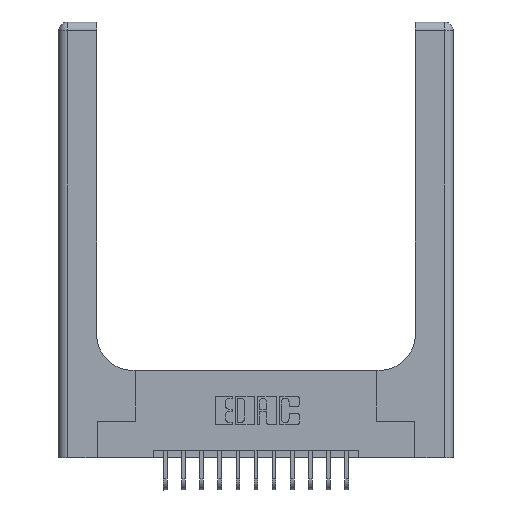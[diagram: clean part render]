
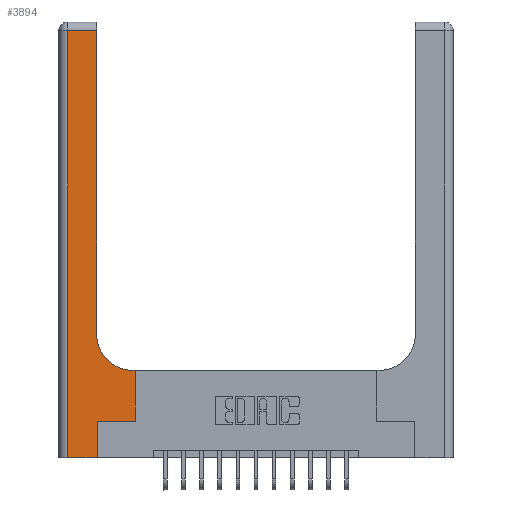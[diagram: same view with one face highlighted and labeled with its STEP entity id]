
A CAD part, top view. The second image highlights one B-rep face of the part: STEP entity #3894.
In plain terms, the highlighted planar face has unit normal (0, 0, 1).
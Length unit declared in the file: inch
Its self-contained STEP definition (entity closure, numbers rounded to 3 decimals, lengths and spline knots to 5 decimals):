
#65 = VECTOR ( 'NONE', #11523, 39.37008 ) ;
#504 = LINE ( 'NONE', #10790, #7117 ) ;
#634 = EDGE_LOOP ( 'NONE', ( #9870, #12955, #15927, #17325, #8818, #16133, #2347, #7431, #12916 ) ) ;
#816 = CARTESIAN_POINT ( 'NONE',  ( 0.06, 2.94, 0.37 ) ) ;
#871 = VECTOR ( 'NONE', #4851, 39.37008 ) ;
#942 = DIRECTION ( 'NONE',  ( 1., 0., 0. ) ) ;
#1199 = EDGE_CURVE ( 'NONE', #12617, #5967, #4763, .T. ) ;
#1299 = VECTOR ( 'NONE', #5661, 39.37008 ) ;
#1865 = DIRECTION ( 'NONE',  ( 0., 0., -1. ) ) ;
#1912 = VECTOR ( 'NONE', #942, 39.37008 ) ;
#2347 = ORIENTED_EDGE ( 'NONE', *, *, #17302, .T. ) ;
#2760 = CIRCLE ( 'NONE', #18224, 0.25 ) ;
#3000 = LINE ( 'NONE', #14559, #1299 ) ;
#3154 = CARTESIAN_POINT ( 'NONE',  ( 0.265, 0., 0.37 ) ) ;
#3252 = LINE ( 'NONE', #4483, #65 ) ;
#3894 = ADVANCED_FACE ( 'NONE', ( #18105 ), #4156, .F. ) ;
#4156 = PLANE ( 'NONE',  #16846 ) ;
#4236 = CARTESIAN_POINT ( 'NONE',  ( 0.26, 0.6, 0.37 ) ) ;
#4483 = CARTESIAN_POINT ( 'NONE',  ( 0.26, 3., 0.37 ) ) ;
#4763 = LINE ( 'NONE', #3154, #871 ) ;
#4851 = DIRECTION ( 'NONE',  ( 0., 1., 0. ) ) ;
#5225 = CARTESIAN_POINT ( 'NONE',  ( 0., 0., 0.37 ) ) ;
#5661 = DIRECTION ( 'NONE',  ( 0., 1., 0. ) ) ;
#5967 = VERTEX_POINT ( 'NONE', #7764 ) ;
#6215 = DIRECTION ( 'NONE',  ( 0., -1., 0. ) ) ;
#6802 = VECTOR ( 'NONE', #13606, 39.37008 ) ;
#7117 = VECTOR ( 'NONE', #6215, 39.37008 ) ;
#7431 = ORIENTED_EDGE ( 'NONE', *, *, #16642, .T. ) ;
#7455 = DIRECTION ( 'NONE',  ( -1., 0., 0. ) ) ;
#7694 = DIRECTION ( 'NONE',  ( 1., 0., 0. ) ) ;
#7743 = CARTESIAN_POINT ( 'NONE',  ( 0.26, 0.85, 0.37 ) ) ;
#7764 = CARTESIAN_POINT ( 'NONE',  ( 0.265, 0.25, 0.37 ) ) ;
#7844 = LINE ( 'NONE', #16715, #6802 ) ;
#8539 = EDGE_CURVE ( 'NONE', #15534, #13504, #2760, .T. ) ;
#8782 = CARTESIAN_POINT ( 'NONE',  ( 0.26, 2.94, 0.37 ) ) ;
#8818 = ORIENTED_EDGE ( 'NONE', *, *, #1199, .T. ) ;
#8916 = LINE ( 'NONE', #4236, #11324 ) ;
#9155 = CARTESIAN_POINT ( 'NONE',  ( 0.528, 0.6, 0.37 ) ) ;
#9666 = EDGE_CURVE ( 'NONE', #13504, #12422, #3252, .T. ) ;
#9870 = ORIENTED_EDGE ( 'NONE', *, *, #9666, .T. ) ;
#9968 = DIRECTION ( 'NONE',  ( -1., 0., 0. ) ) ;
#10422 = LINE ( 'NONE', #14636, #11344 ) ;
#10790 = CARTESIAN_POINT ( 'NONE',  ( 0.06, 3., 0.37 ) ) ;
#10801 = CARTESIAN_POINT ( 'NONE',  ( 0.06, 0., 0.37 ) ) ;
#11324 = VECTOR ( 'NONE', #9968, 39.37008 ) ;
#11344 = VECTOR ( 'NONE', #7455, 39.37008 ) ;
#11455 = CARTESIAN_POINT ( 'NONE',  ( 0., 3., 0.37 ) ) ;
#11523 = DIRECTION ( 'NONE',  ( 0., 1., 0. ) ) ;
#12422 = VERTEX_POINT ( 'NONE', #8782 ) ;
#12516 = EDGE_CURVE ( 'NONE', #18749, #14619, #504, .T. ) ;
#12617 = VERTEX_POINT ( 'NONE', #16916 ) ;
#12916 = ORIENTED_EDGE ( 'NONE', *, *, #8539, .T. ) ;
#12955 = ORIENTED_EDGE ( 'NONE', *, *, #15622, .T. ) ;
#13058 = CARTESIAN_POINT ( 'NONE',  ( 0.528, 0.25, 0.37 ) ) ;
#13504 = VERTEX_POINT ( 'NONE', #7743 ) ;
#13606 = DIRECTION ( 'NONE',  ( 1., 0., 0. ) ) ;
#14559 = CARTESIAN_POINT ( 'NONE',  ( 0.528, 0.25, 0.37 ) ) ;
#14619 = VERTEX_POINT ( 'NONE', #10801 ) ;
#14636 = CARTESIAN_POINT ( 'NONE',  ( 0., 2.94, 0.37 ) ) ;
#14881 = CARTESIAN_POINT ( 'NONE',  ( 0.51, 0.85, 0.37 ) ) ;
#15026 = VERTEX_POINT ( 'NONE', #9155 ) ;
#15089 = LINE ( 'NONE', #5225, #1912 ) ;
#15432 = CARTESIAN_POINT ( 'NONE',  ( 0.51, 0.6, 0.37 ) ) ;
#15477 = EDGE_CURVE ( 'NONE', #14619, #12617, #15089, .T. ) ;
#15534 = VERTEX_POINT ( 'NONE', #15432 ) ;
#15622 = EDGE_CURVE ( 'NONE', #12422, #18749, #10422, .T. ) ;
#15927 = ORIENTED_EDGE ( 'NONE', *, *, #12516, .T. ) ;
#16133 = ORIENTED_EDGE ( 'NONE', *, *, #18007, .T. ) ;
#16642 = EDGE_CURVE ( 'NONE', #15026, #15534, #8916, .T. ) ;
#16715 = CARTESIAN_POINT ( 'NONE',  ( 0.265, 0.25, 0.37 ) ) ;
#16731 = VERTEX_POINT ( 'NONE', #13058 ) ;
#16846 = AXIS2_PLACEMENT_3D ( 'NONE', #11455, #18580, #18762 ) ;
#16916 = CARTESIAN_POINT ( 'NONE',  ( 0.265, 0., 0.37 ) ) ;
#17302 = EDGE_CURVE ( 'NONE', #16731, #15026, #3000, .T. ) ;
#17325 = ORIENTED_EDGE ( 'NONE', *, *, #15477, .T. ) ;
#18007 = EDGE_CURVE ( 'NONE', #5967, #16731, #7844, .T. ) ;
#18105 = FACE_OUTER_BOUND ( 'NONE', #634, .T. ) ;
#18224 = AXIS2_PLACEMENT_3D ( 'NONE', #14881, #1865, #7694 ) ;
#18580 = DIRECTION ( 'NONE',  ( 0., 0., -1. ) ) ;
#18749 = VERTEX_POINT ( 'NONE', #816 ) ;
#18762 = DIRECTION ( 'NONE',  ( -1., 0., 0. ) ) ;
